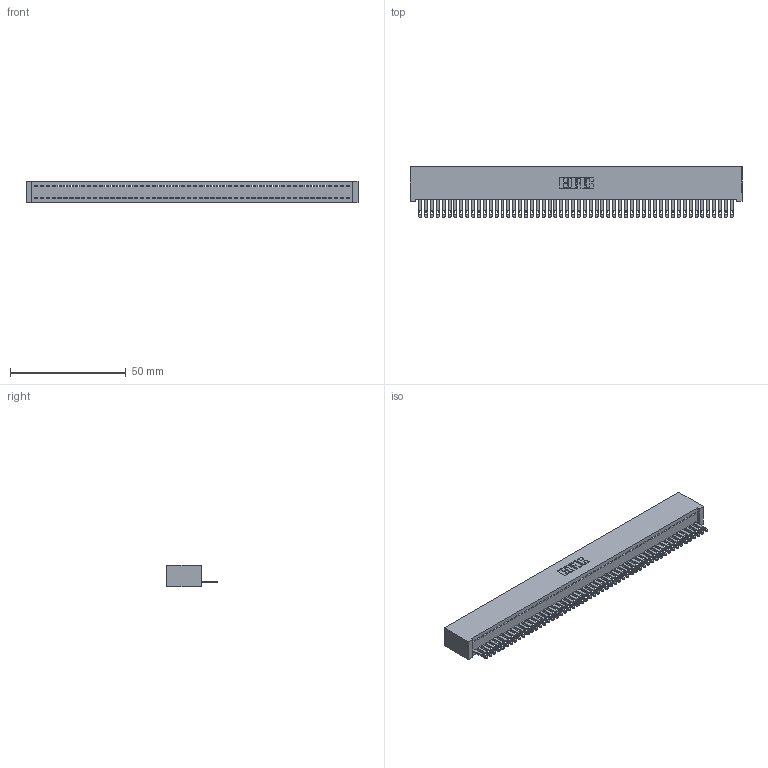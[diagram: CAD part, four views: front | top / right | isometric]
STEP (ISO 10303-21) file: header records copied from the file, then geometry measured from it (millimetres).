
FILE_DESCRIPTION (( 'STEP AP203' ), '1' );
FILE_NAME ('342-054-500-101.STEP', '2018-08-12T23:30:55', ( '' ), ( '' ), 'SwSTEP 2.0', 'SolidWorks 2016', '' );
FILE_SCHEMA (( 'CONFIG_CONTROL_DESIGN' ));
Length unit declared in the file: inch
Products named in the file (3): 345-292-001_345-293-100; 342-054-500-101; 342 Part_Lugless
Assembly tree (55 placements, depth 2):
  342-054-500-101
    342 Part_Lugless
    345-292-001_345-293-100  x54
Bounding box: 143.41 x 21.85 x 9.4 mm (x, y, z)
Volume: 13060.6 mm3; surface area: 19832.6 mm2
Topology: 55 solids, 55 shells, 3018 faces, 9347 edges, 6230 vertices
Faces by surface type: plane 2006, cylinder 1012
Entity records: 30981 total; most frequent: CARTESIAN_POINT 5348, ORIENTED_EDGE 5338, DIRECTION 4481, EDGE_CURVE 2669, VECTOR 2545, LINE 2545, VERTEX_POINT 1778, AXIS2_PLACEMENT_3D 968
